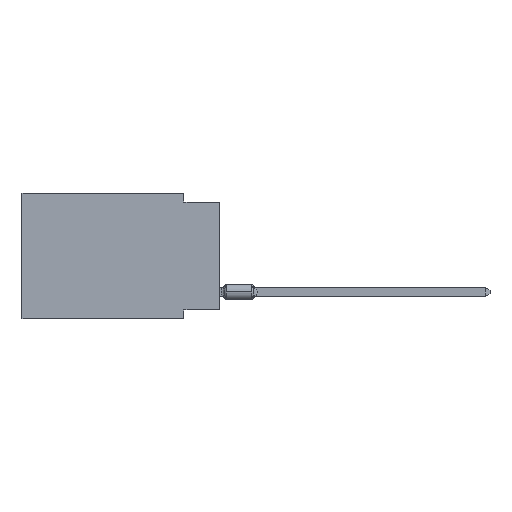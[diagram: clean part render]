
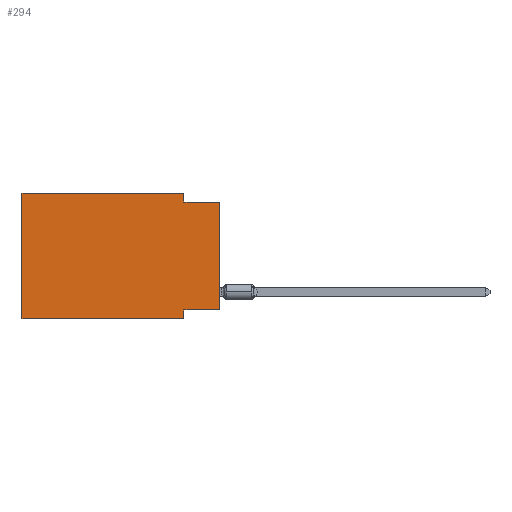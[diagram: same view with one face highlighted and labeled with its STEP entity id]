
A CAD part, left-side view. The second image highlights one B-rep face of the part: STEP entity #294.
In plain terms, the highlighted planar face has unit normal (-1, 0, 0).
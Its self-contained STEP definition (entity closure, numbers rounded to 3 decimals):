
#275 = CARTESIAN_POINT ( 'NONE',  ( 0., 0., 0. ) ) ;
#294 = ADVANCED_FACE ( 'NONE', ( #7625 ), #22209, .F. ) ;
#3323 = CARTESIAN_POINT ( 'NONE',  ( 0., 2.54, -8.89 ) ) ;
#3644 = VECTOR ( 'NONE', #22919, 1000. ) ;
#4303 = VERTEX_POINT ( 'NONE', #19740 ) ;
#5305 = DIRECTION ( 'NONE',  ( 0., -1., 0. ) ) ;
#6378 = ORIENTED_EDGE ( 'NONE', *, *, #20132, .T. ) ;
#6600 = ORIENTED_EDGE ( 'NONE', *, *, #10854, .F. ) ;
#6647 = CARTESIAN_POINT ( 'NONE',  ( 0., 2.54, 0. ) ) ;
#7140 = LINE ( 'NONE', #13020, #10753 ) ;
#7212 = CARTESIAN_POINT ( 'NONE',  ( 0., 13.97, -8.89 ) ) ;
#7357 = VERTEX_POINT ( 'NONE', #7787 ) ;
#7564 = VERTEX_POINT ( 'NONE', #7212 ) ;
#7625 = FACE_OUTER_BOUND ( 'NONE', #11231, .T. ) ;
#7766 = ORIENTED_EDGE ( 'NONE', *, *, #11428, .F. ) ;
#7787 = CARTESIAN_POINT ( 'NONE',  ( 0., 0., -8.255 ) ) ;
#8089 = EDGE_CURVE ( 'NONE', #12778, #22738, #10748, .T. ) ;
#8567 = DIRECTION ( 'NONE',  ( 0., 0., 1. ) ) ;
#8696 = LINE ( 'NONE', #275, #15446 ) ;
#8768 = VECTOR ( 'NONE', #24637, 1000. ) ;
#8966 = DIRECTION ( 'NONE',  ( 0., 0., -1. ) ) ;
#9185 = DIRECTION ( 'NONE',  ( 0., 0., -1. ) ) ;
#9287 = CARTESIAN_POINT ( 'NONE',  ( 0., 13.97, 0. ) ) ;
#10748 = LINE ( 'NONE', #6647, #16934 ) ;
#10753 = VECTOR ( 'NONE', #11118, 1000. ) ;
#10831 = ORIENTED_EDGE ( 'NONE', *, *, #17565, .F. ) ;
#10854 = EDGE_CURVE ( 'NONE', #15249, #25605, #15597, .T. ) ;
#11118 = DIRECTION ( 'NONE',  ( 0., 0., 1. ) ) ;
#11231 = EDGE_LOOP ( 'NONE', ( #11605, #10831, #18839, #7766, #13922, #6378, #6600, #11507 ) ) ;
#11428 = EDGE_CURVE ( 'NONE', #4303, #12778, #13925, .T. ) ;
#11507 = ORIENTED_EDGE ( 'NONE', *, *, #23860, .F. ) ;
#11605 = ORIENTED_EDGE ( 'NONE', *, *, #26403, .T. ) ;
#12778 = VERTEX_POINT ( 'NONE', #15123 ) ;
#12882 = CARTESIAN_POINT ( 'NONE',  ( 0., 2.54, -8.89 ) ) ;
#13020 = CARTESIAN_POINT ( 'NONE',  ( 0., 13.97, 0. ) ) ;
#13060 = EDGE_CURVE ( 'NONE', #7564, #4303, #7140, .T. ) ;
#13502 = DIRECTION ( 'NONE',  ( 0., 0., -1. ) ) ;
#13639 = DIRECTION ( 'NONE',  ( 1., 0., 0. ) ) ;
#13894 = CARTESIAN_POINT ( 'NONE',  ( 0., 0., -0.635 ) ) ;
#13922 = ORIENTED_EDGE ( 'NONE', *, *, #13060, .F. ) ;
#13925 = LINE ( 'NONE', #9287, #21949 ) ;
#15123 = CARTESIAN_POINT ( 'NONE',  ( 0., 2.54, 0. ) ) ;
#15249 = VERTEX_POINT ( 'NONE', #22721 ) ;
#15418 = VECTOR ( 'NONE', #9185, 1000. ) ;
#15446 = VECTOR ( 'NONE', #8567, 1000. ) ;
#15544 = CARTESIAN_POINT ( 'NONE',  ( 0., 13.97, 0. ) ) ;
#15597 = LINE ( 'NONE', #12882, #15418 ) ;
#16387 = CARTESIAN_POINT ( 'NONE',  ( 0., 0., -8.255 ) ) ;
#16637 = AXIS2_PLACEMENT_3D ( 'NONE', #15544, #13639, #13502 ) ;
#16934 = VECTOR ( 'NONE', #8966, 1000. ) ;
#17565 = EDGE_CURVE ( 'NONE', #22738, #22539, #24240, .T. ) ;
#17616 = DIRECTION ( 'NONE',  ( 0., -1., 0. ) ) ;
#18387 = CARTESIAN_POINT ( 'NONE',  ( 0., 13.97, -8.89 ) ) ;
#18798 = LINE ( 'NONE', #18387, #8768 ) ;
#18839 = ORIENTED_EDGE ( 'NONE', *, *, #8089, .F. ) ;
#19740 = CARTESIAN_POINT ( 'NONE',  ( 0., 13.97, 0. ) ) ;
#20132 = EDGE_CURVE ( 'NONE', #7564, #25605, #18798, .T. ) ;
#21138 = CARTESIAN_POINT ( 'NONE',  ( 0., 2.54, -0.635 ) ) ;
#21847 = CARTESIAN_POINT ( 'NONE',  ( 0., 0., -0.635 ) ) ;
#21949 = VECTOR ( 'NONE', #17616, 1000. ) ;
#22209 = PLANE ( 'NONE',  #16637 ) ;
#22539 = VERTEX_POINT ( 'NONE', #21847 ) ;
#22721 = CARTESIAN_POINT ( 'NONE',  ( 0., 2.54, -8.255 ) ) ;
#22738 = VERTEX_POINT ( 'NONE', #21138 ) ;
#22919 = DIRECTION ( 'NONE',  ( 0., 1., 0. ) ) ;
#23860 = EDGE_CURVE ( 'NONE', #7357, #15249, #24948, .T. ) ;
#24240 = LINE ( 'NONE', #13894, #26084 ) ;
#24637 = DIRECTION ( 'NONE',  ( 0., -1., 0. ) ) ;
#24948 = LINE ( 'NONE', #16387, #3644 ) ;
#25605 = VERTEX_POINT ( 'NONE', #3323 ) ;
#26084 = VECTOR ( 'NONE', #5305, 1000. ) ;
#26403 = EDGE_CURVE ( 'NONE', #7357, #22539, #8696, .T. ) ;
